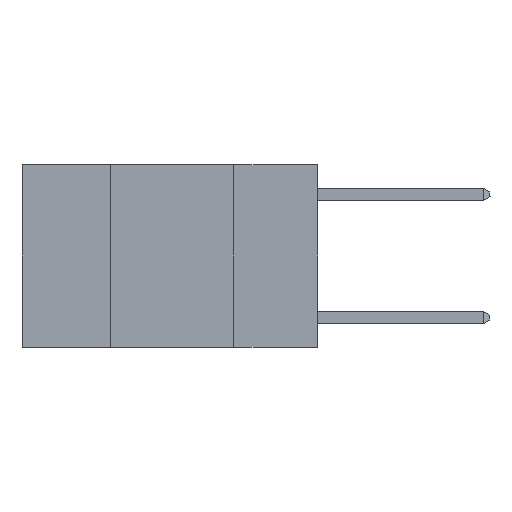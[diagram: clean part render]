
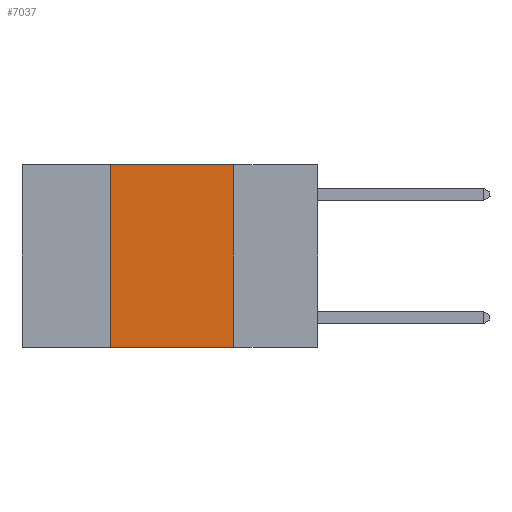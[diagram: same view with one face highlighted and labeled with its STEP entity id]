
A CAD part, left-side view. The second image highlights one B-rep face of the part: STEP entity #7037.
In plain terms, the highlighted planar face has unit normal (-1, 0, 0).
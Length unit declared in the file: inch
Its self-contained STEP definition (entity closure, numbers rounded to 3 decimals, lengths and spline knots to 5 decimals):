
#622 = DIRECTION ( 'NONE',  ( 0., 0., -1. ) ) ;
#1488 = CARTESIAN_POINT ( 'NONE',  ( 0., 0.17, 0. ) ) ;
#2106 = CARTESIAN_POINT ( 'NONE',  ( 0., 0.6, 0. ) ) ;
#2171 = ORIENTED_EDGE ( 'NONE', *, *, #2572, .F. ) ;
#2572 = EDGE_CURVE ( 'NONE', #6689, #17134, #14385, .T. ) ;
#2766 = LINE ( 'NONE', #14646, #17254 ) ;
#3361 = VECTOR ( 'NONE', #17262, 39.37008 ) ;
#3987 = VERTEX_POINT ( 'NONE', #6298 ) ;
#4308 = EDGE_CURVE ( 'NONE', #18643, #17134, #2766, .T. ) ;
#6298 = CARTESIAN_POINT ( 'NONE',  ( 0., 0.42, 0. ) ) ;
#6489 = FACE_OUTER_BOUND ( 'NONE', #17929, .T. ) ;
#6689 = VERTEX_POINT ( 'NONE', #1488 ) ;
#6710 = DIRECTION ( 'NONE',  ( 0., 0., -1. ) ) ;
#7037 = ADVANCED_FACE ( 'NONE', ( #6489 ), #21396, .F. ) ;
#9524 = VECTOR ( 'NONE', #22724, 39.37008 ) ;
#9929 = EDGE_CURVE ( 'NONE', #3987, #6689, #14625, .T. ) ;
#9957 = VECTOR ( 'NONE', #6710, 39.37008 ) ;
#10112 = LINE ( 'NONE', #22564, #9524 ) ;
#10158 = CARTESIAN_POINT ( 'NONE',  ( 0., 0.6, 0. ) ) ;
#12041 = DIRECTION ( 'NONE',  ( 1., 0., 0. ) ) ;
#12210 = CARTESIAN_POINT ( 'NONE',  ( 0., 0.42, -0.37 ) ) ;
#12389 = CARTESIAN_POINT ( 'NONE',  ( 0., 0.17, 0. ) ) ;
#14385 = LINE ( 'NONE', #12389, #9957 ) ;
#14625 = LINE ( 'NONE', #2106, #3361 ) ;
#14646 = CARTESIAN_POINT ( 'NONE',  ( 0., 0.6, -0.37 ) ) ;
#15794 = AXIS2_PLACEMENT_3D ( 'NONE', #10158, #12041, #622 ) ;
#17134 = VERTEX_POINT ( 'NONE', #19740 ) ;
#17254 = VECTOR ( 'NONE', #22186, 39.37008 ) ;
#17262 = DIRECTION ( 'NONE',  ( 0., -1., 0. ) ) ;
#17929 = EDGE_LOOP ( 'NONE', ( #2171, #21698, #21535, #20156 ) ) ;
#18643 = VERTEX_POINT ( 'NONE', #12210 ) ;
#19740 = CARTESIAN_POINT ( 'NONE',  ( 0., 0.17, -0.37 ) ) ;
#20156 = ORIENTED_EDGE ( 'NONE', *, *, #4308, .T. ) ;
#21396 = PLANE ( 'NONE',  #15794 ) ;
#21535 = ORIENTED_EDGE ( 'NONE', *, *, #23718, .F. ) ;
#21698 = ORIENTED_EDGE ( 'NONE', *, *, #9929, .F. ) ;
#22186 = DIRECTION ( 'NONE',  ( 0., -1., 0. ) ) ;
#22564 = CARTESIAN_POINT ( 'NONE',  ( 0., 0.42, 0. ) ) ;
#22724 = DIRECTION ( 'NONE',  ( 0., 0., 1. ) ) ;
#23718 = EDGE_CURVE ( 'NONE', #18643, #3987, #10112, .T. ) ;
